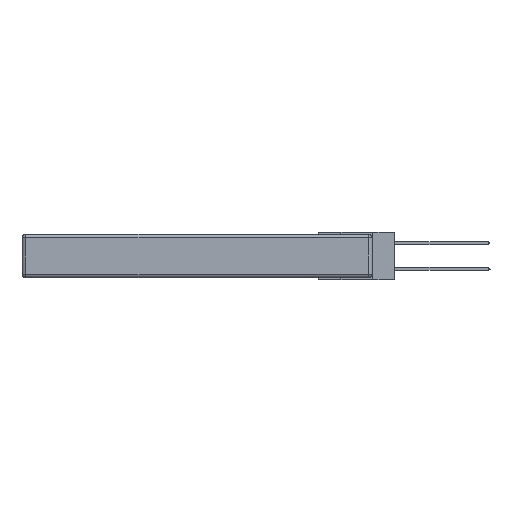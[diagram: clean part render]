
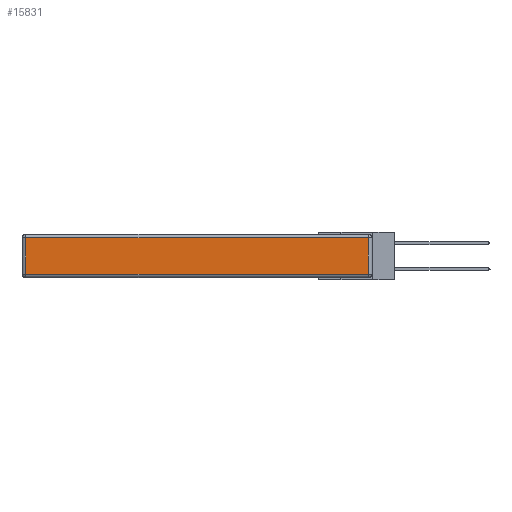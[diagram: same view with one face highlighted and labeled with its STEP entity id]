
A CAD part, left-side view. The second image highlights one B-rep face of the part: STEP entity #15831.
In plain terms, the highlighted planar face has unit normal (-1, 0, 0).
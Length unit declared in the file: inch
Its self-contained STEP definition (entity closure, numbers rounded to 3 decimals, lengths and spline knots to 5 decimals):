
#451 = ORIENTED_EDGE ( 'NONE', *, *, #1708, .T. ) ;
#773 = CARTESIAN_POINT ( 'NONE',  ( 0., 0.03, -0.343 ) ) ;
#1246 = DIRECTION ( 'NONE',  ( 0., 0., -1. ) ) ;
#1708 = EDGE_CURVE ( 'NONE', #20516, #9294, #4072, .T. ) ;
#2486 = VECTOR ( 'NONE', #7330, 39.37008 ) ;
#2926 = CARTESIAN_POINT ( 'NONE',  ( 0., 0.03, -0.313 ) ) ;
#2960 = EDGE_CURVE ( 'NONE', #9294, #4870, #3317, .T. ) ;
#3317 = LINE ( 'NONE', #17926, #23741 ) ;
#4072 = LINE ( 'NONE', #773, #8200 ) ;
#4870 = VERTEX_POINT ( 'NONE', #22539 ) ;
#5000 = DIRECTION ( 'NONE',  ( 0., 1., 0. ) ) ;
#5260 = CARTESIAN_POINT ( 'NONE',  ( 0., 0., -0.313 ) ) ;
#5378 = DIRECTION ( 'NONE',  ( 0., 0., 1. ) ) ;
#5428 = EDGE_LOOP ( 'NONE', ( #23906, #451, #20285, #17482 ) ) ;
#7330 = DIRECTION ( 'NONE',  ( 0., -1., 0. ) ) ;
#8200 = VECTOR ( 'NONE', #10196, 39.37008 ) ;
#9294 = VERTEX_POINT ( 'NONE', #16240 ) ;
#10196 = DIRECTION ( 'NONE',  ( 0., 0., 1. ) ) ;
#12499 = CARTESIAN_POINT ( 'NONE',  ( 0., 2.72, -0.343 ) ) ;
#12574 = PLANE ( 'NONE',  #15263 ) ;
#12910 = CARTESIAN_POINT ( 'NONE',  ( 0., 2.72, -0.313 ) ) ;
#14558 = CARTESIAN_POINT ( 'NONE',  ( 0., 0., -0.343 ) ) ;
#15263 = AXIS2_PLACEMENT_3D ( 'NONE', #14558, #22124, #5378 ) ;
#15760 = EDGE_CURVE ( 'NONE', #4870, #21344, #17719, .T. ) ;
#15831 = ADVANCED_FACE ( 'NONE', ( #17991 ), #12574, .T. ) ;
#16240 = CARTESIAN_POINT ( 'NONE',  ( 0., 0.03, -0.03 ) ) ;
#17482 = ORIENTED_EDGE ( 'NONE', *, *, #15760, .T. ) ;
#17719 = LINE ( 'NONE', #12499, #22479 ) ;
#17926 = CARTESIAN_POINT ( 'NONE',  ( 0., 2.75, -0.03 ) ) ;
#17991 = FACE_OUTER_BOUND ( 'NONE', #5428, .T. ) ;
#18228 = EDGE_CURVE ( 'NONE', #21344, #20516, #21137, .T. ) ;
#20285 = ORIENTED_EDGE ( 'NONE', *, *, #2960, .T. ) ;
#20516 = VERTEX_POINT ( 'NONE', #2926 ) ;
#21137 = LINE ( 'NONE', #5260, #2486 ) ;
#21344 = VERTEX_POINT ( 'NONE', #12910 ) ;
#22124 = DIRECTION ( 'NONE',  ( -1., 0., 0. ) ) ;
#22479 = VECTOR ( 'NONE', #1246, 39.37008 ) ;
#22539 = CARTESIAN_POINT ( 'NONE',  ( 0., 2.72, -0.03 ) ) ;
#23741 = VECTOR ( 'NONE', #5000, 39.37008 ) ;
#23906 = ORIENTED_EDGE ( 'NONE', *, *, #18228, .T. ) ;
